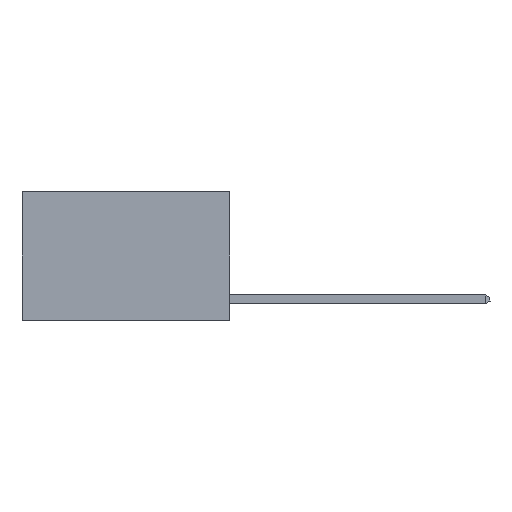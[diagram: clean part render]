
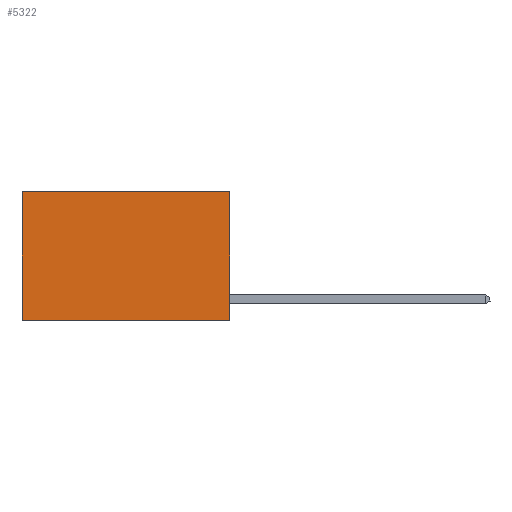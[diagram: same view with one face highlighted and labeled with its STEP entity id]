
A CAD part, left-side view. The second image highlights one B-rep face of the part: STEP entity #5322.
In plain terms, the highlighted planar face has unit normal (-1, 0, 0).
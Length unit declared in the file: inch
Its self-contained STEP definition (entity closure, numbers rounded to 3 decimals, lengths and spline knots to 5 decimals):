
#231 = CARTESIAN_POINT ( 'NONE',  ( 0.2625, 0., -0.37 ) ) ;
#236 = CARTESIAN_POINT ( 'NONE',  ( 0.2625, 0., 0. ) ) ;
#1228 = LINE ( 'NONE', #2444, #3186 ) ;
#2076 = AXIS2_PLACEMENT_3D ( 'NONE', #6891, #10685, #6983 ) ;
#2350 = ORIENTED_EDGE ( 'NONE', *, *, #11923, .T. ) ;
#2444 = CARTESIAN_POINT ( 'NONE',  ( 0.2625, 0., 0. ) ) ;
#3103 = DIRECTION ( 'NONE',  ( 0., 1., 0. ) ) ;
#3150 = ORIENTED_EDGE ( 'NONE', *, *, #10876, .T. ) ;
#3186 = VECTOR ( 'NONE', #4822, 39.37008 ) ;
#3822 = VERTEX_POINT ( 'NONE', #5787 ) ;
#4560 = VERTEX_POINT ( 'NONE', #6158 ) ;
#4822 = DIRECTION ( 'NONE',  ( 0., 1., 0. ) ) ;
#4837 = EDGE_CURVE ( 'NONE', #10978, #10245, #8517, .T. ) ;
#5222 = EDGE_LOOP ( 'NONE', ( #3150, #8190, #8252, #2350 ) ) ;
#5322 = ADVANCED_FACE ( 'NONE', ( #10408 ), #11561, .F. ) ;
#5787 = CARTESIAN_POINT ( 'NONE',  ( 0.2625, 0., 0. ) ) ;
#6153 = CARTESIAN_POINT ( 'NONE',  ( 0.2625, 0.6, 0. ) ) ;
#6158 = CARTESIAN_POINT ( 'NONE',  ( 0.2625, 0.6, 0. ) ) ;
#6617 = EDGE_CURVE ( 'NONE', #3822, #10978, #11293, .T. ) ;
#6859 = DIRECTION ( 'NONE',  ( 0., 0., -1. ) ) ;
#6891 = CARTESIAN_POINT ( 'NONE',  ( 0.2625, 0., 0. ) ) ;
#6983 = DIRECTION ( 'NONE',  ( 0., 0., -1. ) ) ;
#7519 = VECTOR ( 'NONE', #3103, 39.37008 ) ;
#8190 = ORIENTED_EDGE ( 'NONE', *, *, #4837, .F. ) ;
#8252 = ORIENTED_EDGE ( 'NONE', *, *, #6617, .F. ) ;
#8507 = VECTOR ( 'NONE', #6859, 39.37008 ) ;
#8517 = LINE ( 'NONE', #231, #7519 ) ;
#9245 = VECTOR ( 'NONE', #10180, 39.37008 ) ;
#9911 = CARTESIAN_POINT ( 'NONE',  ( 0.2625, 0.6, -0.37 ) ) ;
#10180 = DIRECTION ( 'NONE',  ( 0., 0., -1. ) ) ;
#10245 = VERTEX_POINT ( 'NONE', #9911 ) ;
#10408 = FACE_OUTER_BOUND ( 'NONE', #5222, .T. ) ;
#10685 = DIRECTION ( 'NONE',  ( 1., 0., 0. ) ) ;
#10693 = LINE ( 'NONE', #6153, #9245 ) ;
#10876 = EDGE_CURVE ( 'NONE', #4560, #10245, #10693, .T. ) ;
#10978 = VERTEX_POINT ( 'NONE', #12020 ) ;
#11293 = LINE ( 'NONE', #236, #8507 ) ;
#11561 = PLANE ( 'NONE',  #2076 ) ;
#11923 = EDGE_CURVE ( 'NONE', #3822, #4560, #1228, .T. ) ;
#12020 = CARTESIAN_POINT ( 'NONE',  ( 0.2625, 0., -0.37 ) ) ;
